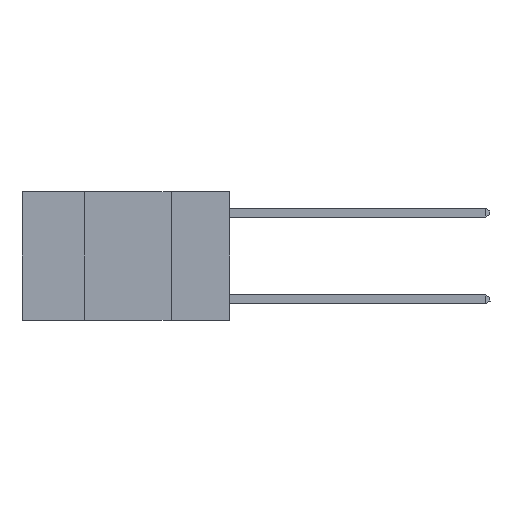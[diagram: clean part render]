
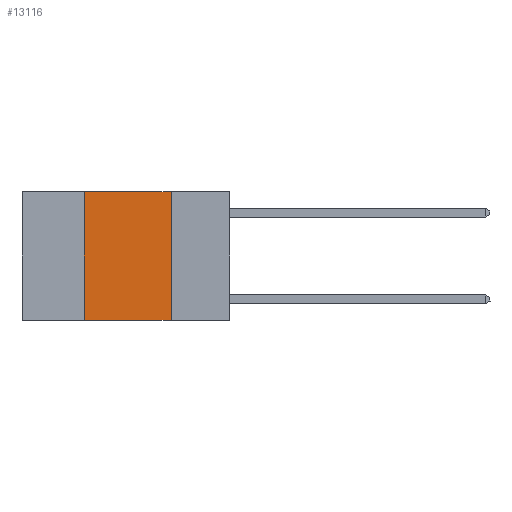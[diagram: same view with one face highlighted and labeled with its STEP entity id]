
A CAD part, left-side view. The second image highlights one B-rep face of the part: STEP entity #13116.
In plain terms, the highlighted planar face has unit normal (-1, 0, 0).
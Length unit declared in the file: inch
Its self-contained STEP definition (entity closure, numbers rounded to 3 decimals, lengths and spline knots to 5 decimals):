
#815 = DIRECTION ( 'NONE',  ( 0., 0., -1. ) ) ;
#1261 = EDGE_CURVE ( 'NONE', #6401, #13726, #11056, .T. ) ;
#1493 = CARTESIAN_POINT ( 'NONE',  ( 0., 0.42, -0.37 ) ) ;
#2645 = ORIENTED_EDGE ( 'NONE', *, *, #3632, .F. ) ;
#2794 = ORIENTED_EDGE ( 'NONE', *, *, #16878, .T. ) ;
#2800 = CARTESIAN_POINT ( 'NONE',  ( 0., 0.6, -0.37 ) ) ;
#2897 = CARTESIAN_POINT ( 'NONE',  ( 0., 0.17, 0. ) ) ;
#3072 = DIRECTION ( 'NONE',  ( 0., 0., 1. ) ) ;
#3607 = PLANE ( 'NONE',  #11567 ) ;
#3632 = EDGE_CURVE ( 'NONE', #13726, #14565, #8616, .T. ) ;
#3701 = DIRECTION ( 'NONE',  ( 1., 0., 0. ) ) ;
#4075 = CARTESIAN_POINT ( 'NONE',  ( 0., 0.6, 0. ) ) ;
#4116 = DIRECTION ( 'NONE',  ( 0., 0., -1. ) ) ;
#4161 = DIRECTION ( 'NONE',  ( 0., -1., 0. ) ) ;
#4510 = VECTOR ( 'NONE', #4161, 39.37008 ) ;
#5522 = VERTEX_POINT ( 'NONE', #1493 ) ;
#5574 = EDGE_CURVE ( 'NONE', #5522, #6401, #7315, .T. ) ;
#5673 = LINE ( 'NONE', #2800, #11815 ) ;
#5963 = EDGE_LOOP ( 'NONE', ( #2645, #6814, #11998, #2794 ) ) ;
#6120 = CARTESIAN_POINT ( 'NONE',  ( 0., 0.42, 0. ) ) ;
#6401 = VERTEX_POINT ( 'NONE', #10935 ) ;
#6814 = ORIENTED_EDGE ( 'NONE', *, *, #1261, .F. ) ;
#7315 = LINE ( 'NONE', #6120, #17236 ) ;
#8616 = LINE ( 'NONE', #2897, #15370 ) ;
#9661 = CARTESIAN_POINT ( 'NONE',  ( 0., 0.17, -0.37 ) ) ;
#10935 = CARTESIAN_POINT ( 'NONE',  ( 0., 0.42, 0. ) ) ;
#11056 = LINE ( 'NONE', #4075, #4510 ) ;
#11567 = AXIS2_PLACEMENT_3D ( 'NONE', #11977, #3701, #815 ) ;
#11815 = VECTOR ( 'NONE', #15196, 39.37008 ) ;
#11977 = CARTESIAN_POINT ( 'NONE',  ( 0., 0.6, 0. ) ) ;
#11998 = ORIENTED_EDGE ( 'NONE', *, *, #5574, .F. ) ;
#12585 = CARTESIAN_POINT ( 'NONE',  ( 0., 0.17, 0. ) ) ;
#13116 = ADVANCED_FACE ( 'NONE', ( #16178 ), #3607, .F. ) ;
#13726 = VERTEX_POINT ( 'NONE', #12585 ) ;
#14565 = VERTEX_POINT ( 'NONE', #9661 ) ;
#15196 = DIRECTION ( 'NONE',  ( 0., -1., 0. ) ) ;
#15370 = VECTOR ( 'NONE', #4116, 39.37008 ) ;
#16178 = FACE_OUTER_BOUND ( 'NONE', #5963, .T. ) ;
#16878 = EDGE_CURVE ( 'NONE', #5522, #14565, #5673, .T. ) ;
#17236 = VECTOR ( 'NONE', #3072, 39.37008 ) ;
